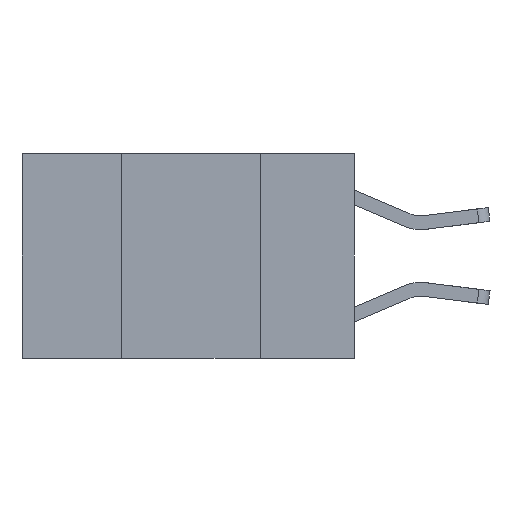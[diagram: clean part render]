
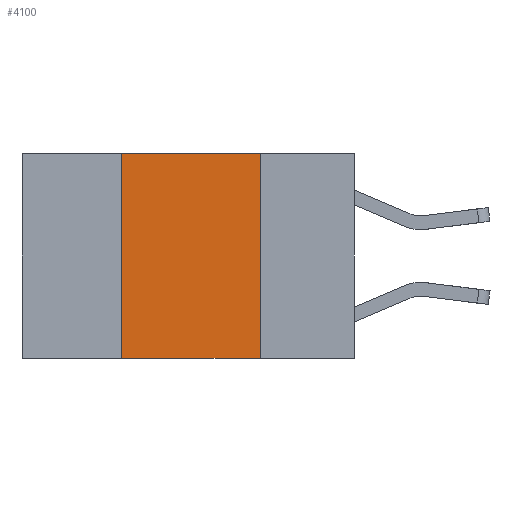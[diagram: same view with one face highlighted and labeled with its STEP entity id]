
A CAD part, left-side view. The second image highlights one B-rep face of the part: STEP entity #4100.
In plain terms, the highlighted planar face has unit normal (-1, 0, 0).
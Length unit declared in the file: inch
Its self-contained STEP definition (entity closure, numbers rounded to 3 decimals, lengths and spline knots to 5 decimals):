
#15 = EDGE_CURVE ( 'NONE', #1821, #8202, #1666, .T. ) ;
#97 = VERTEX_POINT ( 'NONE', #5532 ) ;
#451 = VECTOR ( 'NONE', #7423, 39.37008 ) ;
#656 = CARTESIAN_POINT ( 'NONE',  ( 0., 0.42, 0. ) ) ;
#1125 = DIRECTION ( 'NONE',  ( 0., -1., 0. ) ) ;
#1157 = LINE ( 'NONE', #7968, #8122 ) ;
#1168 = DIRECTION ( 'NONE',  ( 1., 0., 0. ) ) ;
#1245 = DIRECTION ( 'NONE',  ( 0., 0., 1. ) ) ;
#1323 = DIRECTION ( 'NONE',  ( 0., 0., -1. ) ) ;
#1438 = EDGE_CURVE ( 'NONE', #2256, #97, #2528, .T. ) ;
#1666 = LINE ( 'NONE', #7789, #5105 ) ;
#1821 = VERTEX_POINT ( 'NONE', #6256 ) ;
#2015 = LINE ( 'NONE', #2697, #7182 ) ;
#2256 = VERTEX_POINT ( 'NONE', #656 ) ;
#2516 = PLANE ( 'NONE',  #2550 ) ;
#2519 = CARTESIAN_POINT ( 'NONE',  ( 0., 0.6, 0. ) ) ;
#2528 = LINE ( 'NONE', #6882, #451 ) ;
#2550 = AXIS2_PLACEMENT_3D ( 'NONE', #2519, #1168, #1323 ) ;
#2697 = CARTESIAN_POINT ( 'NONE',  ( 0., 0.17, 0. ) ) ;
#4100 = ADVANCED_FACE ( 'NONE', ( #4334 ), #2516, .F. ) ;
#4334 = FACE_OUTER_BOUND ( 'NONE', #5184, .T. ) ;
#4566 = CARTESIAN_POINT ( 'NONE',  ( 0., 0.17, -0.37 ) ) ;
#4699 = EDGE_CURVE ( 'NONE', #1821, #2256, #1157, .T. ) ;
#5105 = VECTOR ( 'NONE', #1125, 39.37008 ) ;
#5184 = EDGE_LOOP ( 'NONE', ( #6940, #8568, #5191, #6313 ) ) ;
#5191 = ORIENTED_EDGE ( 'NONE', *, *, #4699, .F. ) ;
#5532 = CARTESIAN_POINT ( 'NONE',  ( 0., 0.17, 0. ) ) ;
#6038 = EDGE_CURVE ( 'NONE', #97, #8202, #2015, .T. ) ;
#6256 = CARTESIAN_POINT ( 'NONE',  ( 0., 0.42, -0.37 ) ) ;
#6313 = ORIENTED_EDGE ( 'NONE', *, *, #15, .T. ) ;
#6882 = CARTESIAN_POINT ( 'NONE',  ( 0., 0.6, 0. ) ) ;
#6940 = ORIENTED_EDGE ( 'NONE', *, *, #6038, .F. ) ;
#7182 = VECTOR ( 'NONE', #8000, 39.37008 ) ;
#7423 = DIRECTION ( 'NONE',  ( 0., -1., 0. ) ) ;
#7789 = CARTESIAN_POINT ( 'NONE',  ( 0., 0.6, -0.37 ) ) ;
#7968 = CARTESIAN_POINT ( 'NONE',  ( 0., 0.42, 0. ) ) ;
#8000 = DIRECTION ( 'NONE',  ( 0., 0., -1. ) ) ;
#8122 = VECTOR ( 'NONE', #1245, 39.37008 ) ;
#8202 = VERTEX_POINT ( 'NONE', #4566 ) ;
#8568 = ORIENTED_EDGE ( 'NONE', *, *, #1438, .F. ) ;
